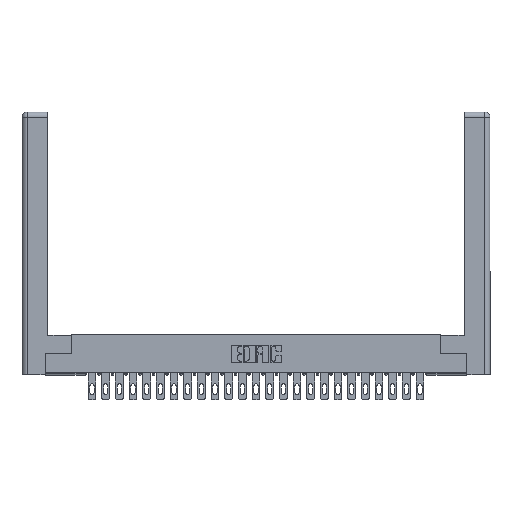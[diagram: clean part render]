
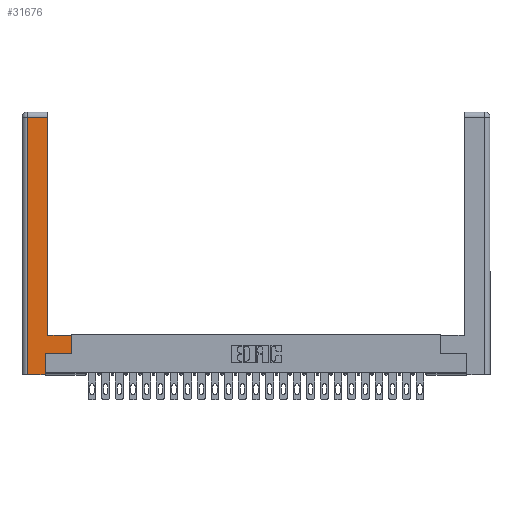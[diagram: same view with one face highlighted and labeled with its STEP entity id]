
A CAD part, top view. The second image highlights one B-rep face of the part: STEP entity #31676.
In plain terms, the highlighted planar face has unit normal (0, 0, 1).
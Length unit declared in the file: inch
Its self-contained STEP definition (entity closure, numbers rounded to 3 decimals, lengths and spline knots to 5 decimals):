
#1896 = VECTOR ( 'NONE', #28030, 39.37008 ) ;
#2049 = CARTESIAN_POINT ( 'NONE',  ( 0.295, 0.45, 0. ) ) ;
#2405 = DIRECTION ( 'NONE',  ( 0., 1., 0. ) ) ;
#3387 = VECTOR ( 'NONE', #2405, 39.37008 ) ;
#3562 = CARTESIAN_POINT ( 'NONE',  ( 0.0615, 2.94, 0. ) ) ;
#3590 = VECTOR ( 'NONE', #15980, 39.37008 ) ;
#3635 = ORIENTED_EDGE ( 'NONE', *, *, #30763, .T. ) ;
#3882 = EDGE_LOOP ( 'NONE', ( #14902, #17297, #19757, #13817, #7840, #7994, #3635, #12024 ) ) ;
#5882 = DIRECTION ( 'NONE',  ( 0., 1., 0. ) ) ;
#5937 = VERTEX_POINT ( 'NONE', #13071 ) ;
#6013 = CARTESIAN_POINT ( 'NONE',  ( 0., 0., 0. ) ) ;
#6773 = DIRECTION ( 'NONE',  ( -1., 0., 0. ) ) ;
#7267 = VECTOR ( 'NONE', #6773, 39.37008 ) ;
#7333 = DIRECTION ( 'NONE',  ( 1., 0., 0. ) ) ;
#7688 = LINE ( 'NONE', #31110, #26573 ) ;
#7840 = ORIENTED_EDGE ( 'NONE', *, *, #26691, .T. ) ;
#7994 = ORIENTED_EDGE ( 'NONE', *, *, #27225, .T. ) ;
#8343 = CARTESIAN_POINT ( 'NONE',  ( 0.565, 0.245, 0. ) ) ;
#9477 = AXIS2_PLACEMENT_3D ( 'NONE', #6013, #25379, #23123 ) ;
#9602 = EDGE_CURVE ( 'NONE', #15893, #19166, #28929, .T. ) ;
#11357 = VERTEX_POINT ( 'NONE', #27660 ) ;
#11638 = CARTESIAN_POINT ( 'NONE',  ( 0.0615, 2.94, 0. ) ) ;
#11659 = LINE ( 'NONE', #13520, #3590 ) ;
#11821 = EDGE_CURVE ( 'NONE', #25462, #15893, #11659, .T. ) ;
#12024 = ORIENTED_EDGE ( 'NONE', *, *, #29493, .T. ) ;
#12093 = CARTESIAN_POINT ( 'NONE',  ( 0.265, 0., 0. ) ) ;
#12128 = EDGE_CURVE ( 'NONE', #18992, #25462, #27060, .T. ) ;
#12754 = CARTESIAN_POINT ( 'NONE',  ( 0.265, 0., 0. ) ) ;
#13071 = CARTESIAN_POINT ( 'NONE',  ( 0.565, 0.45, 0. ) ) ;
#13173 = VECTOR ( 'NONE', #29164, 39.37008 ) ;
#13520 = CARTESIAN_POINT ( 'NONE',  ( 0.0615, 0., 0. ) ) ;
#13817 = ORIENTED_EDGE ( 'NONE', *, *, #9602, .T. ) ;
#14572 = LINE ( 'NONE', #2049, #7267 ) ;
#14582 = LINE ( 'NONE', #8343, #1896 ) ;
#14785 = CARTESIAN_POINT ( 'NONE',  ( 0.0615, 0., 0. ) ) ;
#14902 = ORIENTED_EDGE ( 'NONE', *, *, #16307, .T. ) ;
#14983 = LINE ( 'NONE', #23346, #17303 ) ;
#15893 = VERTEX_POINT ( 'NONE', #14785 ) ;
#15980 = DIRECTION ( 'NONE',  ( 0., -1., 0. ) ) ;
#16307 = EDGE_CURVE ( 'NONE', #11357, #18992, #7688, .T. ) ;
#16373 = DIRECTION ( 'NONE',  ( 0., 1., 0. ) ) ;
#17297 = ORIENTED_EDGE ( 'NONE', *, *, #12128, .T. ) ;
#17303 = VECTOR ( 'NONE', #5882, 39.37008 ) ;
#17371 = VECTOR ( 'NONE', #7333, 39.37008 ) ;
#17372 = CARTESIAN_POINT ( 'NONE',  ( 0.265, 0.245, 0. ) ) ;
#18477 = PLANE ( 'NONE',  #9477 ) ;
#18900 = VERTEX_POINT ( 'NONE', #17372 ) ;
#18992 = VERTEX_POINT ( 'NONE', #29321 ) ;
#19166 = VERTEX_POINT ( 'NONE', #12754 ) ;
#19757 = ORIENTED_EDGE ( 'NONE', *, *, #11821, .T. ) ;
#21467 = LINE ( 'NONE', #29175, #3387 ) ;
#23123 = DIRECTION ( 'NONE',  ( -1., 0., 0. ) ) ;
#23346 = CARTESIAN_POINT ( 'NONE',  ( 0.265, 0.245, 0. ) ) ;
#25379 = DIRECTION ( 'NONE',  ( 0., 0., -1. ) ) ;
#25462 = VERTEX_POINT ( 'NONE', #3562 ) ;
#26573 = VECTOR ( 'NONE', #16373, 39.37008 ) ;
#26691 = EDGE_CURVE ( 'NONE', #19166, #18900, #14983, .T. ) ;
#27060 = LINE ( 'NONE', #11638, #13173 ) ;
#27225 = EDGE_CURVE ( 'NONE', #18900, #31209, #14582, .T. ) ;
#27660 = CARTESIAN_POINT ( 'NONE',  ( 0.295, 0.45, 0. ) ) ;
#28030 = DIRECTION ( 'NONE',  ( 1., 0., 0. ) ) ;
#28200 = CARTESIAN_POINT ( 'NONE',  ( 0.565, 0.245, 0. ) ) ;
#28929 = LINE ( 'NONE', #12093, #17371 ) ;
#29164 = DIRECTION ( 'NONE',  ( -1., 0., 0. ) ) ;
#29175 = CARTESIAN_POINT ( 'NONE',  ( 0.565, 0.45, 0. ) ) ;
#29321 = CARTESIAN_POINT ( 'NONE',  ( 0.295, 2.94, 0. ) ) ;
#29475 = FACE_OUTER_BOUND ( 'NONE', #3882, .T. ) ;
#29493 = EDGE_CURVE ( 'NONE', #5937, #11357, #14572, .T. ) ;
#30763 = EDGE_CURVE ( 'NONE', #31209, #5937, #21467, .T. ) ;
#31110 = CARTESIAN_POINT ( 'NONE',  ( 0.295, 3., 0. ) ) ;
#31209 = VERTEX_POINT ( 'NONE', #28200 ) ;
#31676 = ADVANCED_FACE ( 'NONE', ( #29475 ), #18477, .F. ) ;
